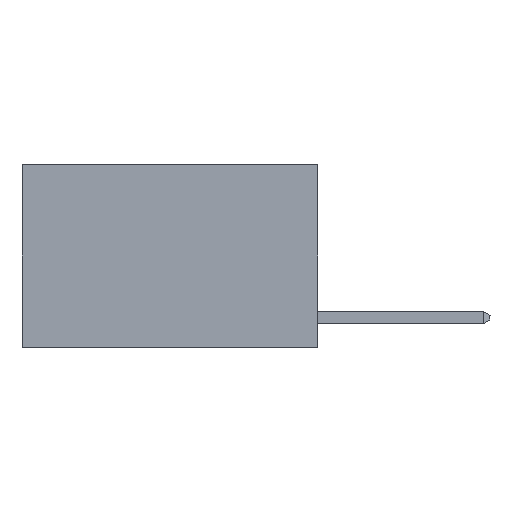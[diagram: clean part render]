
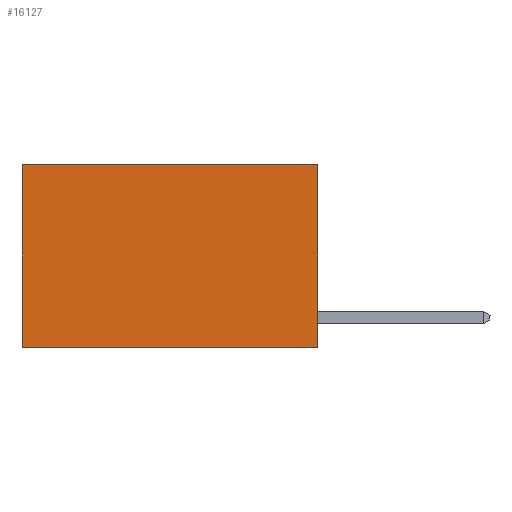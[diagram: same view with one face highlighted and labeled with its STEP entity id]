
A CAD part, left-side view. The second image highlights one B-rep face of the part: STEP entity #16127.
In plain terms, the highlighted planar face has unit normal (-1, 0, 0).
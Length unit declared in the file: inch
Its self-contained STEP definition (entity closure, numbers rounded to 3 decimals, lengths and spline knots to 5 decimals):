
#707 = EDGE_CURVE ( 'NONE', #20192, #18633, #13905, .T. ) ;
#747 = ORIENTED_EDGE ( 'NONE', *, *, #22816, .F. ) ;
#1803 = VERTEX_POINT ( 'NONE', #19165 ) ;
#2808 = VECTOR ( 'NONE', #3830, 39.37008 ) ;
#3830 = DIRECTION ( 'NONE',  ( 0., 0., -1. ) ) ;
#4071 = ORIENTED_EDGE ( 'NONE', *, *, #707, .T. ) ;
#5702 = CARTESIAN_POINT ( 'NONE',  ( 0.2625, 0., 0. ) ) ;
#6132 = PLANE ( 'NONE',  #21692 ) ;
#7499 = DIRECTION ( 'NONE',  ( 0., 0., -1. ) ) ;
#8282 = CARTESIAN_POINT ( 'NONE',  ( 0.2625, 0.6, -0.37 ) ) ;
#8759 = CARTESIAN_POINT ( 'NONE',  ( 0.2625, 0., -0.37 ) ) ;
#10408 = EDGE_CURVE ( 'NONE', #20192, #1803, #15049, .T. ) ;
#10568 = FACE_OUTER_BOUND ( 'NONE', #21642, .T. ) ;
#12071 = LINE ( 'NONE', #21113, #27576 ) ;
#12806 = EDGE_CURVE ( 'NONE', #18633, #21337, #12071, .T. ) ;
#13905 = LINE ( 'NONE', #18352, #14756 ) ;
#14756 = VECTOR ( 'NONE', #22650, 39.37008 ) ;
#15049 = LINE ( 'NONE', #15490, #2808 ) ;
#15288 = DIRECTION ( 'NONE',  ( 0., 0., -1. ) ) ;
#15490 = CARTESIAN_POINT ( 'NONE',  ( 0.2625, 0., 0. ) ) ;
#15555 = DIRECTION ( 'NONE',  ( 0., 1., 0. ) ) ;
#15613 = VECTOR ( 'NONE', #15555, 39.37008 ) ;
#16127 = ADVANCED_FACE ( 'NONE', ( #10568 ), #6132, .F. ) ;
#16261 = ORIENTED_EDGE ( 'NONE', *, *, #12806, .T. ) ;
#17513 = DIRECTION ( 'NONE',  ( 1., 0., 0. ) ) ;
#18352 = CARTESIAN_POINT ( 'NONE',  ( 0.2625, 0., 0. ) ) ;
#18633 = VERTEX_POINT ( 'NONE', #26598 ) ;
#19165 = CARTESIAN_POINT ( 'NONE',  ( 0.2625, 0., -0.37 ) ) ;
#20192 = VERTEX_POINT ( 'NONE', #23902 ) ;
#21113 = CARTESIAN_POINT ( 'NONE',  ( 0.2625, 0.6, 0. ) ) ;
#21337 = VERTEX_POINT ( 'NONE', #8282 ) ;
#21642 = EDGE_LOOP ( 'NONE', ( #16261, #747, #28633, #4071 ) ) ;
#21692 = AXIS2_PLACEMENT_3D ( 'NONE', #5702, #17513, #15288 ) ;
#22650 = DIRECTION ( 'NONE',  ( 0., 1., 0. ) ) ;
#22816 = EDGE_CURVE ( 'NONE', #1803, #21337, #26685, .T. ) ;
#23902 = CARTESIAN_POINT ( 'NONE',  ( 0.2625, 0., 0. ) ) ;
#26598 = CARTESIAN_POINT ( 'NONE',  ( 0.2625, 0.6, 0. ) ) ;
#26685 = LINE ( 'NONE', #8759, #15613 ) ;
#27576 = VECTOR ( 'NONE', #7499, 39.37008 ) ;
#28633 = ORIENTED_EDGE ( 'NONE', *, *, #10408, .F. ) ;
